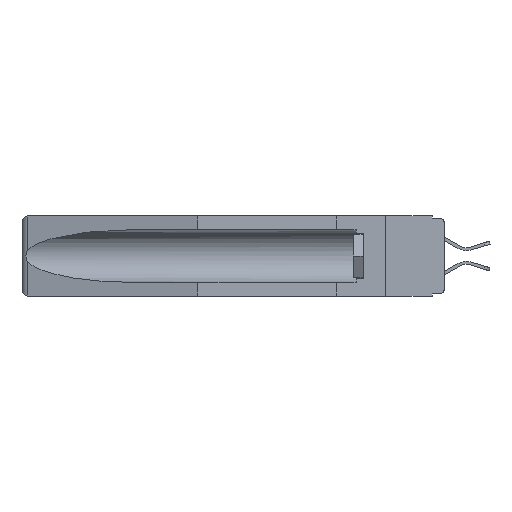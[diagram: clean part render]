
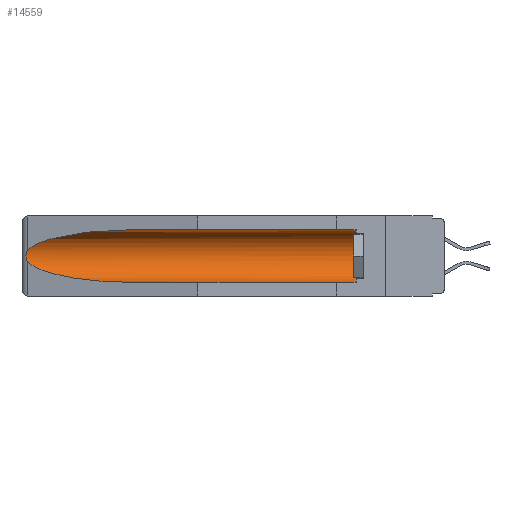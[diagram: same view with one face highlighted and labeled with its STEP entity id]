
A CAD part, left-side view. The second image highlights one B-rep face of the part: STEP entity #14559.
In plain terms, the highlighted cylindrical face has radius 2.857 mm (diameter 5.715 mm), a partial arc.
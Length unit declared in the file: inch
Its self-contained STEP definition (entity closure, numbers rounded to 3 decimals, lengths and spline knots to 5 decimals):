
#145 = EDGE_CURVE ( 'NONE', #21356, #7333, #5270, .T. ) ;
#730 = CARTESIAN_POINT ( 'NONE',  ( 0.155, 1.07973, -0.284 ) ) ;
#960 = EDGE_CURVE ( 'NONE', #21356, #13764, #20089, .T. ) ;
#1013 = CARTESIAN_POINT ( 'NONE',  ( 0.26537, 1.52718, -0.14972 ) ) ;
#1261 = CARTESIAN_POINT ( 'NONE',  ( 0.2673, 1.5327, -0.16383 ) ) ;
#1317 = DIRECTION ( 'NONE',  ( 0., 1., 0. ) ) ;
#1499 = ORIENTED_EDGE ( 'NONE', *, *, #145, .T. ) ;
#1772 = CARTESIAN_POINT ( 'NONE',  ( 0.26537, 1.52718, -0.14972 ) ) ;
#4853 = CARTESIAN_POINT ( 'NONE',  ( 0.155, 0.126, -0.059 ) ) ;
#5119 = CARTESIAN_POINT ( 'NONE',  ( 0.26655, 1.53094, -0.18657 ) ) ;
#5270 = CIRCLE ( 'NONE', #8442, 0.1125 ) ;
#5291 = CARTESIAN_POINT ( 'NONE',  ( 0.155, 1.07973, -0.059 ) ) ;
#5345 = DIRECTION ( 'NONE',  ( 0., 0., 1. ) ) ;
#5582 = AXIS2_PLACEMENT_3D ( 'NONE', #15644, #10133, #6151 ) ;
#6151 = DIRECTION ( 'NONE',  ( 0., 0., 1. ) ) ;
#6469 = EDGE_CURVE ( 'NONE', #22594, #9606, #10249, .T. ) ;
#7060 =( BOUNDED_CURVE ( )  B_SPLINE_CURVE ( 3, ( #13228, #16949, #7476, #15104 ),
 .UNSPECIFIED., .F., .T. ) 
 B_SPLINE_CURVE_WITH_KNOTS ( ( 4, 4 ),
 ( 0.1948, 1.5708 ),
 .UNSPECIFIED. ) 
 CURVE ( )  GEOMETRIC_REPRESENTATION_ITEM ( )  RATIONAL_B_SPLINE_CURVE ( ( 1., 0.848, 0.848, 1. ) ) 
 REPRESENTATION_ITEM ( '' )  );
#7176 = ORIENTED_EDGE ( 'NONE', *, *, #22430, .T. ) ;
#7333 = VERTEX_POINT ( 'NONE', #4853 ) ;
#7476 = CARTESIAN_POINT ( 'NONE',  ( 0.21114, 1.30732, -0.284 ) ) ;
#7796 = ORIENTED_EDGE ( 'NONE', *, *, #960, .F. ) ;
#8442 = AXIS2_PLACEMENT_3D ( 'NONE', #14838, #22409, #5345 ) ;
#8602 = CARTESIAN_POINT ( 'NONE',  ( 0.2675, 1.53308, -0.16763 ) ) ;
#8857 = CARTESIAN_POINT ( 'NONE',  ( 0.26597, 1.52961, -0.15275 ) ) ;
#9606 = VERTEX_POINT ( 'NONE', #1772 ) ;
#10133 = DIRECTION ( 'NONE',  ( 0., 1., 0. ) ) ;
#10249 =( BOUNDED_CURVE ( )  B_SPLINE_CURVE ( 3, ( #5291, #22105, #14533, #22231 ),
 .UNSPECIFIED., .F., .T. ) 
 B_SPLINE_CURVE_WITH_KNOTS ( ( 4, 4 ),
 ( 4.71239, 6.08839 ),
 .UNSPECIFIED. ) 
 CURVE ( )  GEOMETRIC_REPRESENTATION_ITEM ( )  RATIONAL_B_SPLINE_CURVE ( ( 1., 0.848, 0.848, 1. ) ) 
 REPRESENTATION_ITEM ( '' )  );
#10357 = CARTESIAN_POINT ( 'NONE',  ( 0.26597, 1.5296, -0.19026 ) ) ;
#10609 = ORIENTED_EDGE ( 'NONE', *, *, #16546, .T. ) ;
#10722 = CARTESIAN_POINT ( 'NONE',  ( 0.26654, 1.53092, -0.15636 ) ) ;
#10739 = CARTESIAN_POINT ( 'NONE',  ( 0.155, -0.30754, -0.284 ) ) ;
#10773 = LINE ( 'NONE', #24478, #13668 ) ;
#11435 = B_SPLINE_CURVE_WITH_KNOTS ( 'NONE', 3,
 ( #1013, #8857, #10722, #1261, #8602, #18214, #14611, #5119, #10357, #12740 ),
 .UNSPECIFIED., .F., .F.,
 ( 4, 2, 2, 2, 4 ),
 ( 0., 0.00029, 0.00058, 0.00087, 0.00117 ),
 .UNSPECIFIED. ) ;
#12740 = CARTESIAN_POINT ( 'NONE',  ( 0.26537, 1.52718, -0.19328 ) ) ;
#13228 = CARTESIAN_POINT ( 'NONE',  ( 0.26537, 1.52718, -0.19328 ) ) ;
#13668 = VECTOR ( 'NONE', #1317, 39.37008 ) ;
#13764 = VERTEX_POINT ( 'NONE', #730 ) ;
#14141 = VECTOR ( 'NONE', #18095, 39.37008 ) ;
#14533 = CARTESIAN_POINT ( 'NONE',  ( 0.25451, 1.48313, -0.09465 ) ) ;
#14559 = ADVANCED_FACE ( 'NONE', ( #23221 ), #19378, .F. ) ;
#14606 = ORIENTED_EDGE ( 'NONE', *, *, #18715, .T. ) ;
#14611 = CARTESIAN_POINT ( 'NONE',  ( 0.2673, 1.53269, -0.17917 ) ) ;
#14838 = CARTESIAN_POINT ( 'NONE',  ( 0.155, 0.126, -0.1715 ) ) ;
#15104 = CARTESIAN_POINT ( 'NONE',  ( 0.155, 1.07973, -0.284 ) ) ;
#15644 = CARTESIAN_POINT ( 'NONE',  ( 0.155, -0.30754, -0.1715 ) ) ;
#16546 = EDGE_CURVE ( 'NONE', #9606, #21857, #11435, .T. ) ;
#16949 = CARTESIAN_POINT ( 'NONE',  ( 0.25451, 1.48313, -0.24835 ) ) ;
#17113 = CARTESIAN_POINT ( 'NONE',  ( 0.26537, 1.52718, -0.19328 ) ) ;
#17888 = ORIENTED_EDGE ( 'NONE', *, *, #6469, .T. ) ;
#18095 = DIRECTION ( 'NONE',  ( 0., 1., 0. ) ) ;
#18214 = CARTESIAN_POINT ( 'NONE',  ( 0.2675, 1.53308, -0.17534 ) ) ;
#18410 = EDGE_LOOP ( 'NONE', ( #17888, #10609, #7176, #7796, #1499, #14606 ) ) ;
#18715 = EDGE_CURVE ( 'NONE', #7333, #22594, #10773, .T. ) ;
#19378 = CYLINDRICAL_SURFACE ( 'NONE', #5582, 0.1125 ) ;
#20089 = LINE ( 'NONE', #10739, #14141 ) ;
#20165 = CARTESIAN_POINT ( 'NONE',  ( 0.155, 0.126, -0.284 ) ) ;
#20414 = CARTESIAN_POINT ( 'NONE',  ( 0.155, 1.07973, -0.059 ) ) ;
#21356 = VERTEX_POINT ( 'NONE', #20165 ) ;
#21857 = VERTEX_POINT ( 'NONE', #17113 ) ;
#22105 = CARTESIAN_POINT ( 'NONE',  ( 0.21114, 1.30732, -0.059 ) ) ;
#22231 = CARTESIAN_POINT ( 'NONE',  ( 0.26537, 1.52718, -0.14972 ) ) ;
#22409 = DIRECTION ( 'NONE',  ( 0., -1., 0. ) ) ;
#22430 = EDGE_CURVE ( 'NONE', #21857, #13764, #7060, .T. ) ;
#22594 = VERTEX_POINT ( 'NONE', #20414 ) ;
#23221 = FACE_OUTER_BOUND ( 'NONE', #18410, .T. ) ;
#24478 = CARTESIAN_POINT ( 'NONE',  ( 0.155, -0.30754, -0.059 ) ) ;
